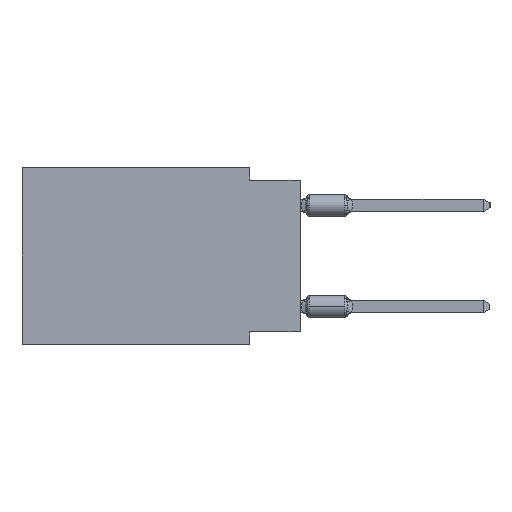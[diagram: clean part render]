
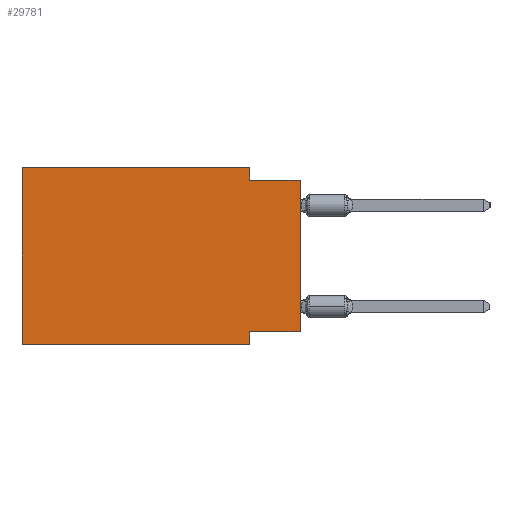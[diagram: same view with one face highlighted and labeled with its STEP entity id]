
A CAD part, left-side view. The second image highlights one B-rep face of the part: STEP entity #29781.
In plain terms, the highlighted planar face has unit normal (-1, 0, 0).
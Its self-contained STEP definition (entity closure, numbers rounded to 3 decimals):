
#260 = DIRECTION ( 'NONE',  ( 0., -1., 0. ) ) ;
#2155 = CARTESIAN_POINT ( 'NONE',  ( 0., 13.97, 0. ) ) ;
#2346 = CARTESIAN_POINT ( 'NONE',  ( 0., 2.54, -0.635 ) ) ;
#2571 = CARTESIAN_POINT ( 'NONE',  ( 0., 13.97, 0. ) ) ;
#2680 = DIRECTION ( 'NONE',  ( 0., -1., 0. ) ) ;
#3797 = VERTEX_POINT ( 'NONE', #13873 ) ;
#3876 = CARTESIAN_POINT ( 'NONE',  ( 0., 0., -8.255 ) ) ;
#4425 = VECTOR ( 'NONE', #18050, 1000. ) ;
#4824 = EDGE_CURVE ( 'NONE', #42576, #16418, #26011, .T. ) ;
#5662 = FACE_OUTER_BOUND ( 'NONE', #18002, .T. ) ;
#6522 = CARTESIAN_POINT ( 'NONE',  ( 0., 0., -8.255 ) ) ;
#6925 = VECTOR ( 'NONE', #15098, 1000. ) ;
#7163 = VERTEX_POINT ( 'NONE', #31446 ) ;
#7543 = VERTEX_POINT ( 'NONE', #9578 ) ;
#7800 = EDGE_CURVE ( 'NONE', #17467, #7543, #42306, .T. ) ;
#9561 = VERTEX_POINT ( 'NONE', #6522 ) ;
#9578 = CARTESIAN_POINT ( 'NONE',  ( 0., 0., -0.635 ) ) ;
#11875 = DIRECTION ( 'NONE',  ( 0., 0., -1. ) ) ;
#12387 = VECTOR ( 'NONE', #39188, 1000. ) ;
#13873 = CARTESIAN_POINT ( 'NONE',  ( 0., 2.54, -8.89 ) ) ;
#14105 = VECTOR ( 'NONE', #260, 1000. ) ;
#14230 = VECTOR ( 'NONE', #11875, 1000. ) ;
#14430 = LINE ( 'NONE', #28612, #34041 ) ;
#15098 = DIRECTION ( 'NONE',  ( 0., -1., 0. ) ) ;
#15115 = CARTESIAN_POINT ( 'NONE',  ( 0., 2.54, -8.89 ) ) ;
#15234 = AXIS2_PLACEMENT_3D ( 'NONE', #2155, #35105, #28380 ) ;
#16418 = VERTEX_POINT ( 'NONE', #25294 ) ;
#16851 = CARTESIAN_POINT ( 'NONE',  ( 0., 13.97, -8.89 ) ) ;
#17467 = VERTEX_POINT ( 'NONE', #2346 ) ;
#17735 = ORIENTED_EDGE ( 'NONE', *, *, #7800, .F. ) ;
#18002 = EDGE_LOOP ( 'NONE', ( #45780, #17735, #30645, #30833, #38704, #29279, #23297, #19060 ) ) ;
#18050 = DIRECTION ( 'NONE',  ( 0., 1., 0. ) ) ;
#18095 = VECTOR ( 'NONE', #2680, 1000. ) ;
#19060 = ORIENTED_EDGE ( 'NONE', *, *, #43247, .F. ) ;
#22584 = EDGE_CURVE ( 'NONE', #9561, #7543, #26931, .T. ) ;
#23297 = ORIENTED_EDGE ( 'NONE', *, *, #25096, .F. ) ;
#25013 = LINE ( 'NONE', #31744, #12387 ) ;
#25096 = EDGE_CURVE ( 'NONE', #7163, #3797, #43697, .T. ) ;
#25294 = CARTESIAN_POINT ( 'NONE',  ( 0., 2.54, 0. ) ) ;
#26011 = LINE ( 'NONE', #32984, #6925 ) ;
#26164 = EDGE_CURVE ( 'NONE', #16418, #17467, #14430, .T. ) ;
#26931 = LINE ( 'NONE', #27618, #31520 ) ;
#27307 = LINE ( 'NONE', #16851, #18095 ) ;
#27322 = CARTESIAN_POINT ( 'NONE',  ( 0., 13.97, -8.89 ) ) ;
#27618 = CARTESIAN_POINT ( 'NONE',  ( 0., 0., 0. ) ) ;
#28380 = DIRECTION ( 'NONE',  ( 0., 0., -1. ) ) ;
#28612 = CARTESIAN_POINT ( 'NONE',  ( 0., 2.54, 0. ) ) ;
#28750 = LINE ( 'NONE', #3876, #4425 ) ;
#29279 = ORIENTED_EDGE ( 'NONE', *, *, #35770, .T. ) ;
#29781 = ADVANCED_FACE ( 'NONE', ( #5662 ), #33981, .F. ) ;
#30636 = DIRECTION ( 'NONE',  ( 0., 0., 1. ) ) ;
#30645 = ORIENTED_EDGE ( 'NONE', *, *, #26164, .F. ) ;
#30833 = ORIENTED_EDGE ( 'NONE', *, *, #4824, .F. ) ;
#31446 = CARTESIAN_POINT ( 'NONE',  ( 0., 2.54, -8.255 ) ) ;
#31520 = VECTOR ( 'NONE', #30636, 1000. ) ;
#31744 = CARTESIAN_POINT ( 'NONE',  ( 0., 13.97, 0. ) ) ;
#31793 = VERTEX_POINT ( 'NONE', #27322 ) ;
#32064 = CARTESIAN_POINT ( 'NONE',  ( 0., 0., -0.635 ) ) ;
#32984 = CARTESIAN_POINT ( 'NONE',  ( 0., 13.97, 0. ) ) ;
#33981 = PLANE ( 'NONE',  #15234 ) ;
#34041 = VECTOR ( 'NONE', #42788, 1000. ) ;
#35105 = DIRECTION ( 'NONE',  ( 1., 0., 0. ) ) ;
#35770 = EDGE_CURVE ( 'NONE', #31793, #3797, #27307, .T. ) ;
#38704 = ORIENTED_EDGE ( 'NONE', *, *, #40383, .F. ) ;
#39188 = DIRECTION ( 'NONE',  ( 0., 0., 1. ) ) ;
#40383 = EDGE_CURVE ( 'NONE', #31793, #42576, #25013, .T. ) ;
#42306 = LINE ( 'NONE', #32064, #14105 ) ;
#42576 = VERTEX_POINT ( 'NONE', #2571 ) ;
#42788 = DIRECTION ( 'NONE',  ( 0., 0., -1. ) ) ;
#43247 = EDGE_CURVE ( 'NONE', #9561, #7163, #28750, .T. ) ;
#43697 = LINE ( 'NONE', #15115, #14230 ) ;
#45780 = ORIENTED_EDGE ( 'NONE', *, *, #22584, .T. ) ;
